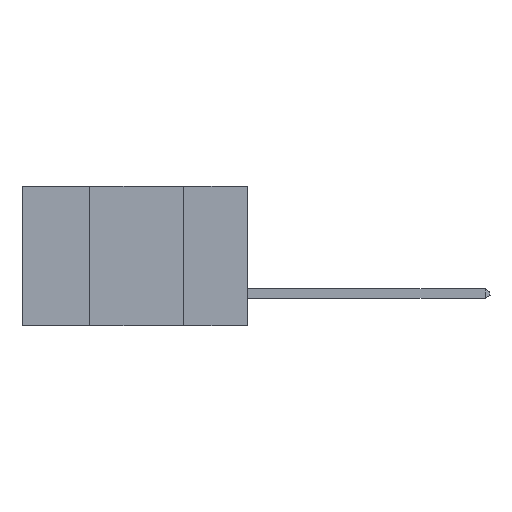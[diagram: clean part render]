
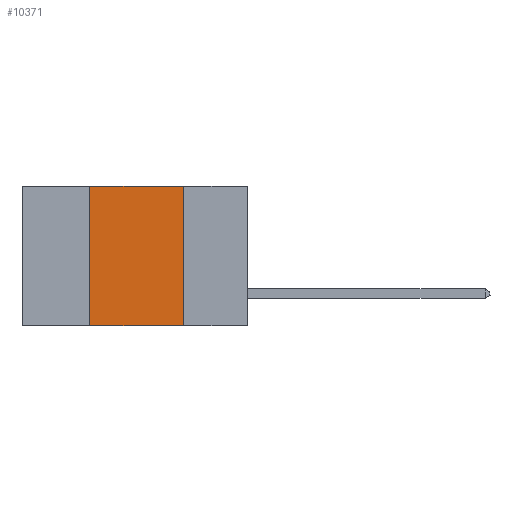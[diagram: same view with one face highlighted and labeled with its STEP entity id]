
A CAD part, left-side view. The second image highlights one B-rep face of the part: STEP entity #10371.
In plain terms, the highlighted planar face has unit normal (-1, 0, 0).
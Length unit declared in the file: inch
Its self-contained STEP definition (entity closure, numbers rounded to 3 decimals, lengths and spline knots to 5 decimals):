
#397 = CARTESIAN_POINT ( 'NONE',  ( 0., 0.6, -0.37 ) ) ;
#836 = CARTESIAN_POINT ( 'NONE',  ( 0., 0.17, 0. ) ) ;
#1010 = ORIENTED_EDGE ( 'NONE', *, *, #8106, .F. ) ;
#1649 = EDGE_CURVE ( 'NONE', #4430, #9669, #2502, .T. ) ;
#1865 = CARTESIAN_POINT ( 'NONE',  ( 0., 0.17, -0.37 ) ) ;
#2502 = LINE ( 'NONE', #13544, #10179 ) ;
#2661 = LINE ( 'NONE', #836, #11038 ) ;
#3269 = CARTESIAN_POINT ( 'NONE',  ( 0., 0.6, 0. ) ) ;
#4182 = EDGE_LOOP ( 'NONE', ( #13121, #9027, #1010, #5810 ) ) ;
#4430 = VERTEX_POINT ( 'NONE', #11423 ) ;
#4443 = DIRECTION ( 'NONE',  ( 0., 0., 1. ) ) ;
#5286 = CARTESIAN_POINT ( 'NONE',  ( 0., 0.42, -0.37 ) ) ;
#5597 = CARTESIAN_POINT ( 'NONE',  ( 0., 0.42, 0. ) ) ;
#5810 = ORIENTED_EDGE ( 'NONE', *, *, #13335, .T. ) ;
#6750 = DIRECTION ( 'NONE',  ( 0., 0., -1. ) ) ;
#6857 = VECTOR ( 'NONE', #4443, 39.37008 ) ;
#7173 = VERTEX_POINT ( 'NONE', #5286 ) ;
#7229 = LINE ( 'NONE', #5597, #6857 ) ;
#7247 = VECTOR ( 'NONE', #12873, 39.37008 ) ;
#7589 = LINE ( 'NONE', #397, #7247 ) ;
#8106 = EDGE_CURVE ( 'NONE', #7173, #4430, #7229, .T. ) ;
#9027 = ORIENTED_EDGE ( 'NONE', *, *, #1649, .F. ) ;
#9669 = VERTEX_POINT ( 'NONE', #12974 ) ;
#9794 = DIRECTION ( 'NONE',  ( 0., 0., -1. ) ) ;
#9960 = DIRECTION ( 'NONE',  ( 0., -1., 0. ) ) ;
#10179 = VECTOR ( 'NONE', #9960, 39.37008 ) ;
#10371 = ADVANCED_FACE ( 'NONE', ( #13930 ), #11305, .F. ) ;
#10677 = VERTEX_POINT ( 'NONE', #1865 ) ;
#11038 = VECTOR ( 'NONE', #9794, 39.37008 ) ;
#11305 = PLANE ( 'NONE',  #11566 ) ;
#11423 = CARTESIAN_POINT ( 'NONE',  ( 0., 0.42, 0. ) ) ;
#11566 = AXIS2_PLACEMENT_3D ( 'NONE', #3269, #13614, #6750 ) ;
#11992 = EDGE_CURVE ( 'NONE', #9669, #10677, #2661, .T. ) ;
#12873 = DIRECTION ( 'NONE',  ( 0., -1., 0. ) ) ;
#12974 = CARTESIAN_POINT ( 'NONE',  ( 0., 0.17, 0. ) ) ;
#13121 = ORIENTED_EDGE ( 'NONE', *, *, #11992, .F. ) ;
#13335 = EDGE_CURVE ( 'NONE', #7173, #10677, #7589, .T. ) ;
#13544 = CARTESIAN_POINT ( 'NONE',  ( 0., 0.6, 0. ) ) ;
#13614 = DIRECTION ( 'NONE',  ( 1., 0., 0. ) ) ;
#13930 = FACE_OUTER_BOUND ( 'NONE', #4182, .T. ) ;
